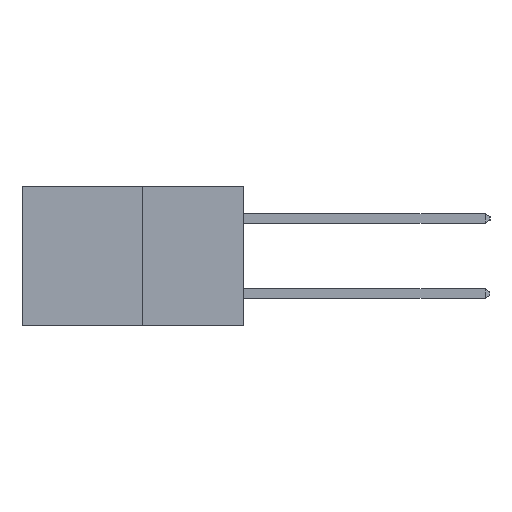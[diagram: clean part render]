
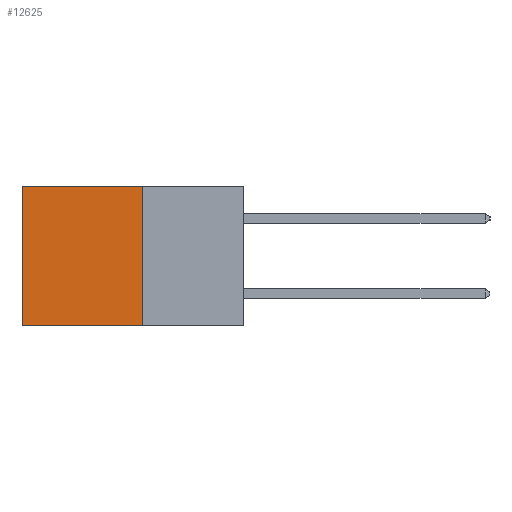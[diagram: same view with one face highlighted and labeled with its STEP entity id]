
A CAD part, left-side view. The second image highlights one B-rep face of the part: STEP entity #12625.
In plain terms, the highlighted planar face has unit normal (-1, 0, 0).
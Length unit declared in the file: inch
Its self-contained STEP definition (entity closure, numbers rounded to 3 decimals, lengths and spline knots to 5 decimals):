
#2184 = DIRECTION ( 'NONE',  ( 1., 0., 0. ) ) ;
#2216 = ORIENTED_EDGE ( 'NONE', *, *, #3591, .T. ) ;
#2237 = VERTEX_POINT ( 'NONE', #22632 ) ;
#2366 = VERTEX_POINT ( 'NONE', #8392 ) ;
#3591 = EDGE_CURVE ( 'NONE', #2237, #14801, #22308, .T. ) ;
#3762 = EDGE_CURVE ( 'NONE', #14801, #18544, #13419, .T. ) ;
#6543 = VECTOR ( 'NONE', #21548, 39.37008 ) ;
#6777 = ORIENTED_EDGE ( 'NONE', *, *, #26635, .F. ) ;
#6788 = ORIENTED_EDGE ( 'NONE', *, *, #20041, .F. ) ;
#8277 = FACE_OUTER_BOUND ( 'NONE', #25829, .T. ) ;
#8312 = AXIS2_PLACEMENT_3D ( 'NONE', #15948, #2184, #18240 ) ;
#8392 = CARTESIAN_POINT ( 'NONE',  ( 0.277, 0.27, -0.37 ) ) ;
#8780 = DIRECTION ( 'NONE',  ( 0., 1., 0. ) ) ;
#9084 = CARTESIAN_POINT ( 'NONE',  ( 0.277, 0.27, -0.37 ) ) ;
#11250 = DIRECTION ( 'NONE',  ( 0., 1., 0. ) ) ;
#12625 = ADVANCED_FACE ( 'NONE', ( #8277 ), #29428, .F. ) ;
#13419 = LINE ( 'NONE', #23284, #6543 ) ;
#13655 = CARTESIAN_POINT ( 'NONE',  ( 0.277, 0.27, 0. ) ) ;
#14622 = VECTOR ( 'NONE', #25025, 39.37008 ) ;
#14801 = VERTEX_POINT ( 'NONE', #27355 ) ;
#15948 = CARTESIAN_POINT ( 'NONE',  ( 0.277, 0.27, -0.37 ) ) ;
#16535 = LINE ( 'NONE', #27168, #27115 ) ;
#17721 = VECTOR ( 'NONE', #8780, 39.37008 ) ;
#18240 = DIRECTION ( 'NONE',  ( 0., 0., -1. ) ) ;
#18544 = VERTEX_POINT ( 'NONE', #24790 ) ;
#20041 = EDGE_CURVE ( 'NONE', #2366, #18544, #16535, .T. ) ;
#21548 = DIRECTION ( 'NONE',  ( 0., 0., -1. ) ) ;
#22308 = LINE ( 'NONE', #13655, #17721 ) ;
#22482 = ORIENTED_EDGE ( 'NONE', *, *, #3762, .T. ) ;
#22632 = CARTESIAN_POINT ( 'NONE',  ( 0.277, 0.27, 0. ) ) ;
#23284 = CARTESIAN_POINT ( 'NONE',  ( 0.277, 0.59, -0.37 ) ) ;
#24790 = CARTESIAN_POINT ( 'NONE',  ( 0.277, 0.59, -0.37 ) ) ;
#25025 = DIRECTION ( 'NONE',  ( 0., 0., -1. ) ) ;
#25829 = EDGE_LOOP ( 'NONE', ( #22482, #6788, #6777, #2216 ) ) ;
#25951 = LINE ( 'NONE', #9084, #14622 ) ;
#26635 = EDGE_CURVE ( 'NONE', #2237, #2366, #25951, .T. ) ;
#27115 = VECTOR ( 'NONE', #11250, 39.37008 ) ;
#27168 = CARTESIAN_POINT ( 'NONE',  ( 0.277, 0.27, -0.37 ) ) ;
#27355 = CARTESIAN_POINT ( 'NONE',  ( 0.277, 0.59, 0. ) ) ;
#29428 = PLANE ( 'NONE',  #8312 ) ;
